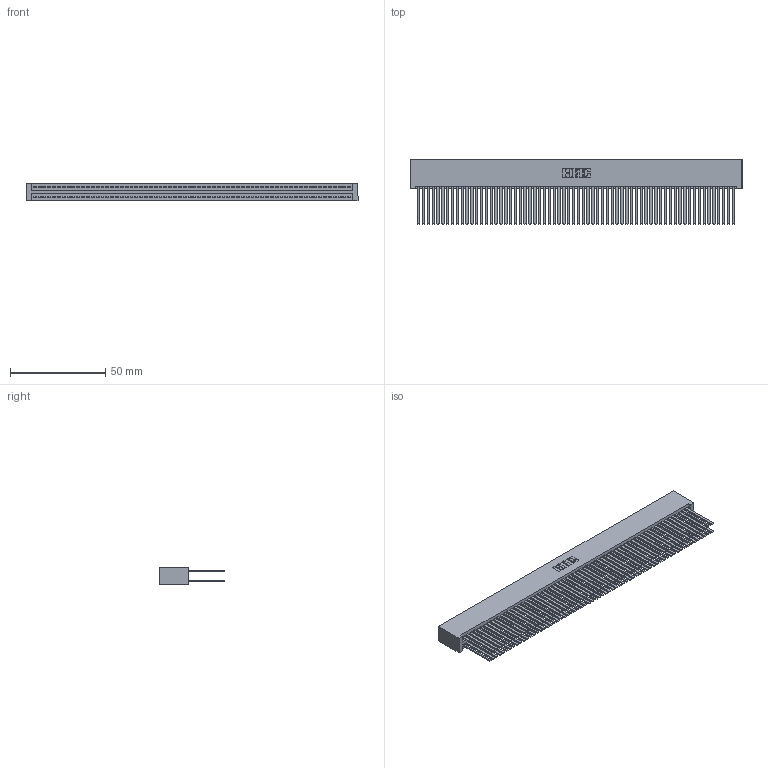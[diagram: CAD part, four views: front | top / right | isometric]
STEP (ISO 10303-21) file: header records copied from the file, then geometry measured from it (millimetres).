
FILE_DESCRIPTION (( 'STEP AP203' ), '1' );
FILE_NAME ('345-132-544-201.STEP', '2018-10-20T05:21:40', ( '' ), ( '' ), 'SwSTEP 2.0', 'SolidWorks 2016', '' );
FILE_SCHEMA (( 'CONFIG_CONTROL_DESIGN' ));
Length unit declared in the file: inch
Products named in the file (3): 345-132-544-201; 345 Part_No Mounting Lugs; 345-292-001_345-293-144
Assembly tree (133 placements, depth 2):
  345-132-544-201
    345 Part_No Mounting Lugs
    345-292-001_345-293-144  x132
Bounding box: 174.24 x 33.96 x 9.4 mm (x, y, z)
Volume: 19615.3 mm3; surface area: 35186.2 mm2
Topology: 133 solids, 133 shells, 5926 faces, 17609 edges, 11562 vertices
Faces by surface type: plane 3904, cylinder 2022
Entity records: 48093 total; most frequent: CARTESIAN_POINT 8036, ORIENTED_EDGE 7970, DIRECTION 7049, EDGE_CURVE 3985, LINE 3601, VECTOR 3601, VERTEX_POINT 2654, AXIS2_PLACEMENT_3D 1724
